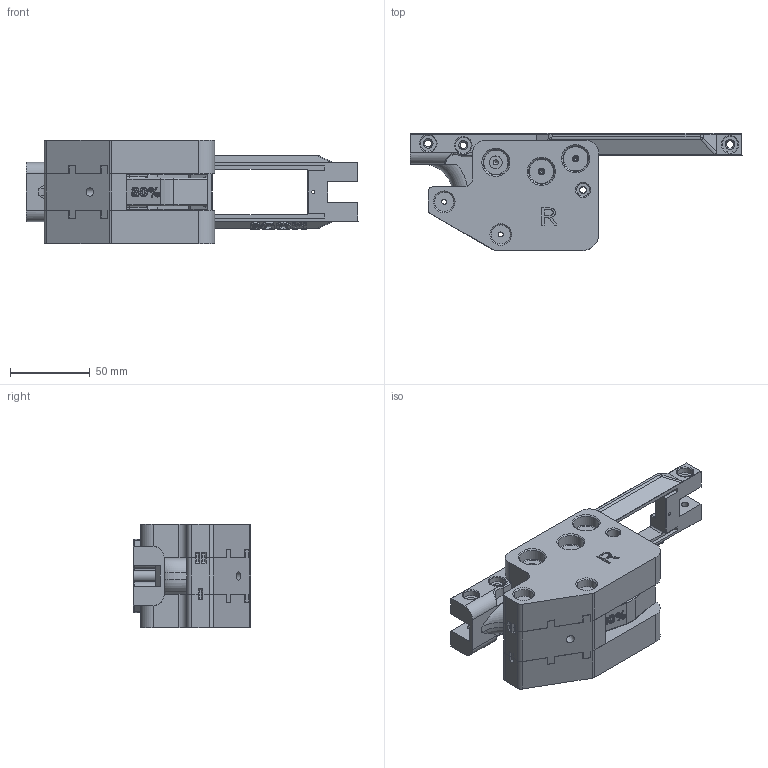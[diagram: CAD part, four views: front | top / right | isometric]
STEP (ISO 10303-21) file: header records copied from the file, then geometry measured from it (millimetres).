
FILE_DESCRIPTION(/* description */ (''),/* implementation_level */ '2;1');
FILE_NAME(/* name */ '80% LOWER AND DRILLING JIG v2.stp',/* time_stamp */ '2020-08-28T13:17:43+03:00',/* author */ (''),/* organization */ (''),/* preprocessor_version */ 'ST-DEVELOPER v15.2',/* originating_system */ 'Autodesk Translator Framework v2.0.0.5431',/* authorisation */ '');
FILE_SCHEMA (('AUTOMOTIVE_DESIGN { 1 0 10303 214 3 1 1 }'));
Products named in the file (1): (Unsaved)
Bounding box: 208.05 x 73.33 x 65.02 mm (x, y, z)
Volume: 357577.7 mm3; surface area: 95918.2 mm2
Topology: 4 solids, 5 shells, 1064 faces, 2750 edges, 1720 vertices
Faces by surface type: bspline 371, plane 341, cylinder 230, torus 62, cone 56, sphere 4
Full cylindrical faces by diameter (mm): 2 x3, 3.1 x6, 3.175 x1, 4 x5, 4.175 x2, 4.4 x2, 4.6 x4, 4.605 x1, 5.305 x1, 8 x4, 10 x6, 12 x4, 16 x6
Entity records: 47653 total; most frequent: CARTESIAN_POINT 24478, ORIENTED_EDGE 5256, DIRECTION 3811, EDGE_CURVE 2627, VERTEX_POINT 1704, AXIS2_PLACEMENT_3D 1299, EDGE_LOOP 1248, LINE 1213
